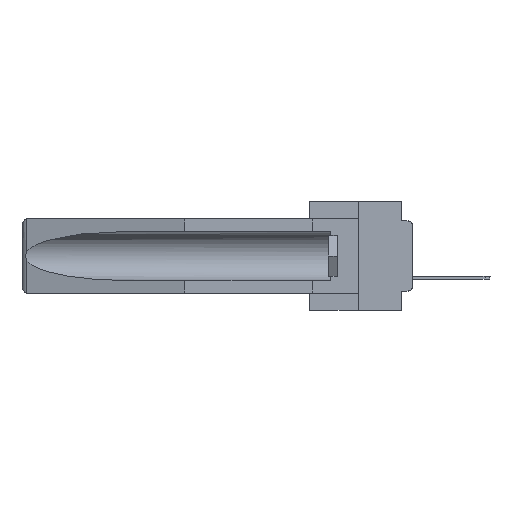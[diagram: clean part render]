
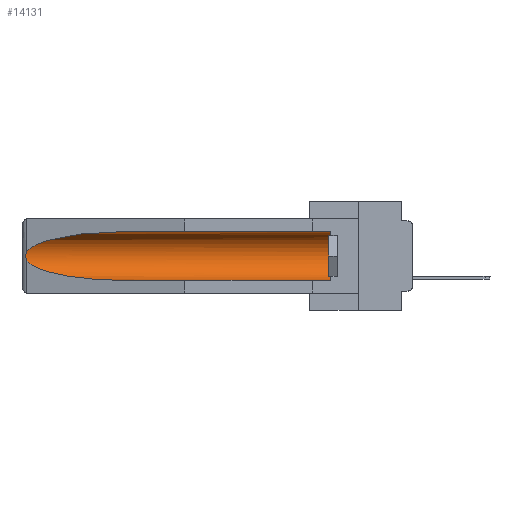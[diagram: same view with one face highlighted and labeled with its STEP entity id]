
A CAD part, left-side view. The second image highlights one B-rep face of the part: STEP entity #14131.
In plain terms, the highlighted cylindrical face has radius 2.857 mm (diameter 5.715 mm), a partial arc.
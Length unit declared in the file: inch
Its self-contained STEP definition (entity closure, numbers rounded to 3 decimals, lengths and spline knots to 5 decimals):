
#306 = DIRECTION ( 'NONE',  ( 0., 0., 1. ) ) ;
#457 = EDGE_CURVE ( 'NONE', #17148, #7369, #22839, .T. ) ;
#1015 = DIRECTION ( 'NONE',  ( 0., 0., 1. ) ) ;
#2970 = CARTESIAN_POINT ( 'NONE',  ( 0.26537, 1.52718, -0.19328 ) ) ;
#3461 = CARTESIAN_POINT ( 'NONE',  ( 0.2673, 1.53269, -0.17917 ) ) ;
#3693 = CARTESIAN_POINT ( 'NONE',  ( 0.155, 0.126, -0.059 ) ) ;
#4020 = CARTESIAN_POINT ( 'NONE',  ( 0.21114, 1.30732, -0.059 ) ) ;
#4091 = ORIENTED_EDGE ( 'NONE', *, *, #8961, .T. ) ;
#4466 = CARTESIAN_POINT ( 'NONE',  ( 0.26537, 1.52718, -0.14972 ) ) ;
#4599 = FACE_OUTER_BOUND ( 'NONE', #10822, .T. ) ;
#5771 = CARTESIAN_POINT ( 'NONE',  ( 0.26597, 1.5296, -0.19026 ) ) ;
#5844 = EDGE_CURVE ( 'NONE', #26683, #19136, #22902, .T. ) ;
#6737 = VERTEX_POINT ( 'NONE', #12198 ) ;
#7136 = B_SPLINE_CURVE_WITH_KNOTS ( 'NONE', 3,
 ( #28812, #26503, #15010, #20043, #17307, #29406, #3461, #29105, #5771, #12562 ),
 .UNSPECIFIED., .F., .F.,
 ( 4, 2, 2, 2, 4 ),
 ( 0., 0.00029, 0.00058, 0.00087, 0.00117 ),
 .UNSPECIFIED. ) ;
#7369 = VERTEX_POINT ( 'NONE', #3693 ) ;
#8129 = LINE ( 'NONE', #8269, #17960 ) ;
#8131 = CARTESIAN_POINT ( 'NONE',  ( 0.26537, 1.52718, -0.19328 ) ) ;
#8269 = CARTESIAN_POINT ( 'NONE',  ( 0.155, -0.30754, -0.284 ) ) ;
#8961 = EDGE_CURVE ( 'NONE', #28834, #6737, #13499, .T. ) ;
#9824 = CARTESIAN_POINT ( 'NONE',  ( 0.155, -0.30754, -0.1715 ) ) ;
#10747 = DIRECTION ( 'NONE',  ( 0., 1., 0. ) ) ;
#10822 = EDGE_LOOP ( 'NONE', ( #30022, #30298, #4091, #22371, #27684, #11457 ) ) ;
#11173 = CARTESIAN_POINT ( 'NONE',  ( 0.26537, 1.52718, -0.14972 ) ) ;
#11457 = ORIENTED_EDGE ( 'NONE', *, *, #20907, .T. ) ;
#11698 = AXIS2_PLACEMENT_3D ( 'NONE', #9824, #19193, #306 ) ;
#12198 = CARTESIAN_POINT ( 'NONE',  ( 0.155, 1.07973, -0.284 ) ) ;
#12562 = CARTESIAN_POINT ( 'NONE',  ( 0.26537, 1.52718, -0.19328 ) ) ;
#13499 =( BOUNDED_CURVE ( )  B_SPLINE_CURVE ( 3, ( #2970, #23694, #23852, #21388 ),
 .UNSPECIFIED., .F., .F. ) 
 B_SPLINE_CURVE_WITH_KNOTS ( ( 4, 4 ),
 ( 0.1948, 1.5708 ),
 .UNSPECIFIED. ) 
 CURVE ( )  GEOMETRIC_REPRESENTATION_ITEM ( )  RATIONAL_B_SPLINE_CURVE ( ( 1., 0.848, 0.848, 1. ) ) 
 REPRESENTATION_ITEM ( '' )  );
#14131 = ADVANCED_FACE ( 'NONE', ( #4599 ), #21479, .F. ) ;
#15010 = CARTESIAN_POINT ( 'NONE',  ( 0.26654, 1.53092, -0.15636 ) ) ;
#16950 = AXIS2_PLACEMENT_3D ( 'NONE', #26650, #22052, #1015 ) ;
#16958 = LINE ( 'NONE', #28299, #19524 ) ;
#17148 = VERTEX_POINT ( 'NONE', #19663 ) ;
#17226 = EDGE_CURVE ( 'NONE', #17148, #6737, #8129, .T. ) ;
#17307 = CARTESIAN_POINT ( 'NONE',  ( 0.2675, 1.53308, -0.16763 ) ) ;
#17960 = VECTOR ( 'NONE', #10747, 39.37008 ) ;
#19136 = VERTEX_POINT ( 'NONE', #11173 ) ;
#19193 = DIRECTION ( 'NONE',  ( 0., 1., 0. ) ) ;
#19524 = VECTOR ( 'NONE', #23848, 39.37008 ) ;
#19663 = CARTESIAN_POINT ( 'NONE',  ( 0.155, 0.126, -0.284 ) ) ;
#20043 = CARTESIAN_POINT ( 'NONE',  ( 0.2673, 1.5327, -0.16383 ) ) ;
#20907 = EDGE_CURVE ( 'NONE', #7369, #26683, #16958, .T. ) ;
#21388 = CARTESIAN_POINT ( 'NONE',  ( 0.155, 1.07973, -0.284 ) ) ;
#21479 = CYLINDRICAL_SURFACE ( 'NONE', #11698, 0.1125 ) ;
#22052 = DIRECTION ( 'NONE',  ( 0., -1., 0. ) ) ;
#22371 = ORIENTED_EDGE ( 'NONE', *, *, #17226, .F. ) ;
#22839 = CIRCLE ( 'NONE', #16950, 0.1125 ) ;
#22902 =( BOUNDED_CURVE ( )  B_SPLINE_CURVE ( 3, ( #27659, #4020, #30113, #4466 ),
 .UNSPECIFIED., .F., .F. ) 
 B_SPLINE_CURVE_WITH_KNOTS ( ( 4, 4 ),
 ( 4.71239, 6.08839 ),
 .UNSPECIFIED. ) 
 CURVE ( )  GEOMETRIC_REPRESENTATION_ITEM ( )  RATIONAL_B_SPLINE_CURVE ( ( 1., 0.848, 0.848, 1. ) ) 
 REPRESENTATION_ITEM ( '' )  );
#23694 = CARTESIAN_POINT ( 'NONE',  ( 0.25451, 1.48313, -0.24835 ) ) ;
#23802 = EDGE_CURVE ( 'NONE', #19136, #28834, #7136, .T. ) ;
#23848 = DIRECTION ( 'NONE',  ( 0., 1., 0. ) ) ;
#23852 = CARTESIAN_POINT ( 'NONE',  ( 0.21114, 1.30732, -0.284 ) ) ;
#26503 = CARTESIAN_POINT ( 'NONE',  ( 0.26597, 1.52961, -0.15275 ) ) ;
#26650 = CARTESIAN_POINT ( 'NONE',  ( 0.155, 0.126, -0.1715 ) ) ;
#26683 = VERTEX_POINT ( 'NONE', #29697 ) ;
#27659 = CARTESIAN_POINT ( 'NONE',  ( 0.155, 1.07973, -0.059 ) ) ;
#27684 = ORIENTED_EDGE ( 'NONE', *, *, #457, .T. ) ;
#28299 = CARTESIAN_POINT ( 'NONE',  ( 0.155, -0.30754, -0.059 ) ) ;
#28812 = CARTESIAN_POINT ( 'NONE',  ( 0.26537, 1.52718, -0.14972 ) ) ;
#28834 = VERTEX_POINT ( 'NONE', #8131 ) ;
#29105 = CARTESIAN_POINT ( 'NONE',  ( 0.26655, 1.53094, -0.18657 ) ) ;
#29406 = CARTESIAN_POINT ( 'NONE',  ( 0.2675, 1.53308, -0.17534 ) ) ;
#29697 = CARTESIAN_POINT ( 'NONE',  ( 0.155, 1.07973, -0.059 ) ) ;
#30022 = ORIENTED_EDGE ( 'NONE', *, *, #5844, .T. ) ;
#30113 = CARTESIAN_POINT ( 'NONE',  ( 0.25451, 1.48313, -0.09465 ) ) ;
#30298 = ORIENTED_EDGE ( 'NONE', *, *, #23802, .T. ) ;
